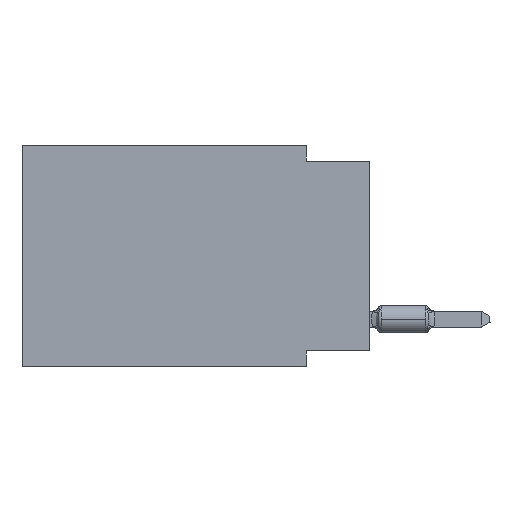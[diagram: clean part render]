
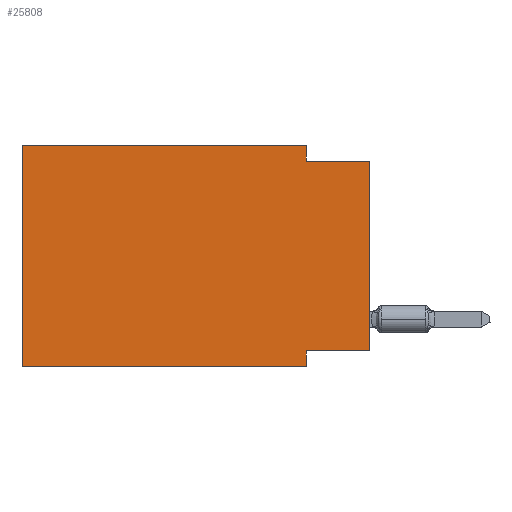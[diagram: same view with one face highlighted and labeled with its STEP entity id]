
A CAD part, left-side view. The second image highlights one B-rep face of the part: STEP entity #25808.
In plain terms, the highlighted planar face has unit normal (-1, 0, 0).
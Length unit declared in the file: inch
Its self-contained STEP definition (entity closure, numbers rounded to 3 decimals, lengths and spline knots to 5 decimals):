
#747 = VECTOR ( 'NONE', #12186, 39.37008 ) ;
#3201 = VECTOR ( 'NONE', #4550, 39.37008 ) ;
#4240 = VERTEX_POINT ( 'NONE', #41897 ) ;
#4550 = DIRECTION ( 'NONE',  ( 0., -1., 0. ) ) ;
#5042 = ORIENTED_EDGE ( 'NONE', *, *, #37118, .F. ) ;
#5576 = PLANE ( 'NONE',  #41269 ) ;
#6005 = VERTEX_POINT ( 'NONE', #38994 ) ;
#6164 = LINE ( 'NONE', #44222, #41693 ) ;
#10163 = CARTESIAN_POINT ( 'NONE',  ( 0., 0.55, 0. ) ) ;
#10194 = DIRECTION ( 'NONE',  ( 0., 0., -1. ) ) ;
#12186 = DIRECTION ( 'NONE',  ( 0., 1., 0. ) ) ;
#12460 = ORIENTED_EDGE ( 'NONE', *, *, #21360, .T. ) ;
#14427 = CARTESIAN_POINT ( 'NONE',  ( 0., 0., -0.025 ) ) ;
#14657 = VERTEX_POINT ( 'NONE', #57176 ) ;
#15329 = EDGE_CURVE ( 'NONE', #4240, #46997, #54695, .T. ) ;
#15605 = EDGE_CURVE ( 'NONE', #46997, #6005, #34171, .T. ) ;
#16720 = CARTESIAN_POINT ( 'NONE',  ( 0., 0.55, -0.35 ) ) ;
#16775 = EDGE_CURVE ( 'NONE', #14657, #19571, #34463, .T. ) ;
#17000 = ORIENTED_EDGE ( 'NONE', *, *, #43351, .F. ) ;
#18371 = VECTOR ( 'NONE', #30788, 39.37008 ) ;
#19571 = VERTEX_POINT ( 'NONE', #33322 ) ;
#20066 = ORIENTED_EDGE ( 'NONE', *, *, #15329, .F. ) ;
#21360 = EDGE_CURVE ( 'NONE', #14657, #36793, #38789, .T. ) ;
#21847 = CARTESIAN_POINT ( 'NONE',  ( 0., 0.55, -0.35 ) ) ;
#25808 = ADVANCED_FACE ( 'NONE', ( #36852 ), #5576, .F. ) ;
#26553 = CARTESIAN_POINT ( 'NONE',  ( 0., 0., -0.025 ) ) ;
#27116 = DIRECTION ( 'NONE',  ( 0., 0., -1. ) ) ;
#27839 = DIRECTION ( 'NONE',  ( 0., -1., 0. ) ) ;
#28438 = DIRECTION ( 'NONE',  ( 1., 0., 0. ) ) ;
#30048 = VERTEX_POINT ( 'NONE', #16720 ) ;
#30069 = DIRECTION ( 'NONE',  ( 0., 0., 1. ) ) ;
#30788 = DIRECTION ( 'NONE',  ( 0., -1., 0. ) ) ;
#33322 = CARTESIAN_POINT ( 'NONE',  ( 0., 0.1, -0.325 ) ) ;
#34171 = LINE ( 'NONE', #38827, #55124 ) ;
#34463 = LINE ( 'NONE', #52103, #747 ) ;
#34568 = EDGE_CURVE ( 'NONE', #30048, #42244, #43842, .T. ) ;
#36566 = CARTESIAN_POINT ( 'NONE',  ( 0., 0.55, 0. ) ) ;
#36793 = VERTEX_POINT ( 'NONE', #14427 ) ;
#36852 = FACE_OUTER_BOUND ( 'NONE', #52732, .T. ) ;
#37118 = EDGE_CURVE ( 'NONE', #19571, #42244, #6164, .T. ) ;
#38789 = LINE ( 'NONE', #56380, #51168 ) ;
#38827 = CARTESIAN_POINT ( 'NONE',  ( 0., 0.1, 0. ) ) ;
#38994 = CARTESIAN_POINT ( 'NONE',  ( 0., 0.1, -0.025 ) ) ;
#40875 = EDGE_CURVE ( 'NONE', #30048, #4240, #44561, .T. ) ;
#41269 = AXIS2_PLACEMENT_3D ( 'NONE', #36566, #28438, #10194 ) ;
#41466 = ORIENTED_EDGE ( 'NONE', *, *, #40875, .F. ) ;
#41693 = VECTOR ( 'NONE', #27116, 39.37008 ) ;
#41897 = CARTESIAN_POINT ( 'NONE',  ( 0., 0.55, 0. ) ) ;
#42219 = VECTOR ( 'NONE', #27839, 39.37008 ) ;
#42244 = VERTEX_POINT ( 'NONE', #43510 ) ;
#43012 = ORIENTED_EDGE ( 'NONE', *, *, #34568, .T. ) ;
#43351 = EDGE_CURVE ( 'NONE', #6005, #36793, #53151, .T. ) ;
#43510 = CARTESIAN_POINT ( 'NONE',  ( 0., 0.1, -0.35 ) ) ;
#43842 = LINE ( 'NONE', #21847, #18371 ) ;
#44222 = CARTESIAN_POINT ( 'NONE',  ( 0., 0.1, -0.35 ) ) ;
#44561 = LINE ( 'NONE', #52924, #44625 ) ;
#44625 = VECTOR ( 'NONE', #47732, 39.37008 ) ;
#46997 = VERTEX_POINT ( 'NONE', #47545 ) ;
#47545 = CARTESIAN_POINT ( 'NONE',  ( 0., 0.1, 0. ) ) ;
#47732 = DIRECTION ( 'NONE',  ( 0., 0., 1. ) ) ;
#51168 = VECTOR ( 'NONE', #30069, 39.37008 ) ;
#52094 = DIRECTION ( 'NONE',  ( 0., 0., -1. ) ) ;
#52103 = CARTESIAN_POINT ( 'NONE',  ( 0., 0., -0.325 ) ) ;
#52732 = EDGE_LOOP ( 'NONE', ( #12460, #17000, #54966, #20066, #41466, #43012, #5042, #56529 ) ) ;
#52924 = CARTESIAN_POINT ( 'NONE',  ( 0., 0.55, 0. ) ) ;
#53151 = LINE ( 'NONE', #26553, #3201 ) ;
#54695 = LINE ( 'NONE', #10163, #42219 ) ;
#54966 = ORIENTED_EDGE ( 'NONE', *, *, #15605, .F. ) ;
#55124 = VECTOR ( 'NONE', #52094, 39.37008 ) ;
#56380 = CARTESIAN_POINT ( 'NONE',  ( 0., 0., 0. ) ) ;
#56529 = ORIENTED_EDGE ( 'NONE', *, *, #16775, .F. ) ;
#57176 = CARTESIAN_POINT ( 'NONE',  ( 0., 0., -0.325 ) ) ;
